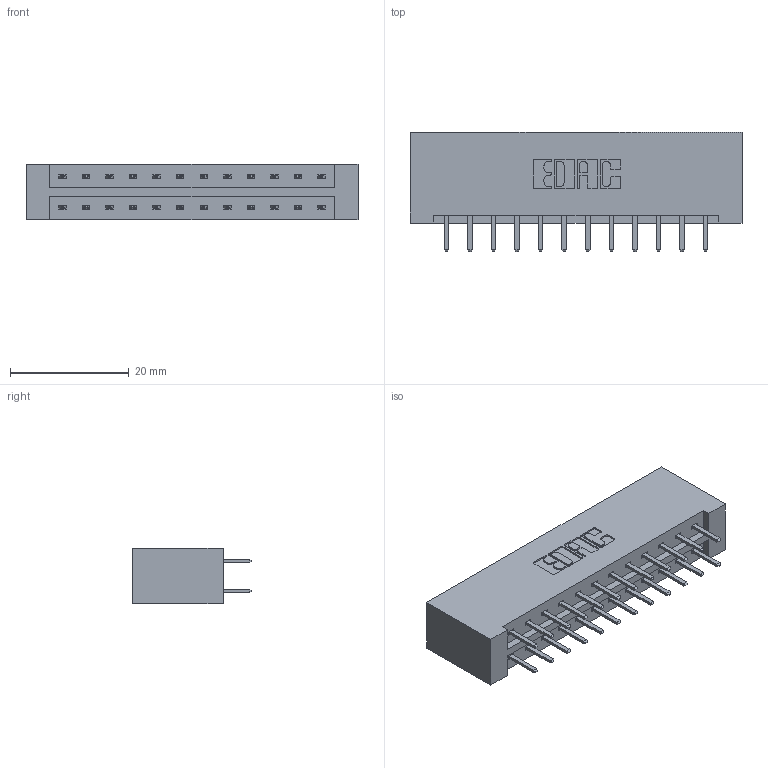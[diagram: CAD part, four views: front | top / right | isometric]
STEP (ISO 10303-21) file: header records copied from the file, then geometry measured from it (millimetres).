
FILE_DESCRIPTION (( 'STEP AP203' ), '1' );
FILE_NAME ('333-024-520-201.STEP', '2018-08-02T04:04:16', ( '' ), ( '' ), 'SwSTEP 2.0', 'SolidWorks 2016', '' );
FILE_SCHEMA (( 'CONFIG_CONTROL_DESIGN' ));
Length unit declared in the file: inch
Products named in the file (3): 333 Part_Lugless; 345-292-001_345-293-120; 333-024-520-201
Assembly tree (25 placements, depth 2):
  333-024-520-201
    333 Part_Lugless
    345-292-001_345-293-120  x24
Bounding box: 55.8 x 20.02 x 9.4 mm (x, y, z)
Volume: 6038.4 mm3; surface area: 6812.9 mm2
Topology: 25 solids, 25 shells, 1450 faces, 4199 edges, 2734 vertices
Faces by surface type: plane 978, cylinder 472
Entity records: 11437 total; most frequent: CARTESIAN_POINT 1942, ORIENTED_EDGE 1866, DIRECTION 1693, EDGE_CURVE 933, VECTOR 809, LINE 809, VERTEX_POINT 618, AXIS2_PLACEMENT_3D 442
